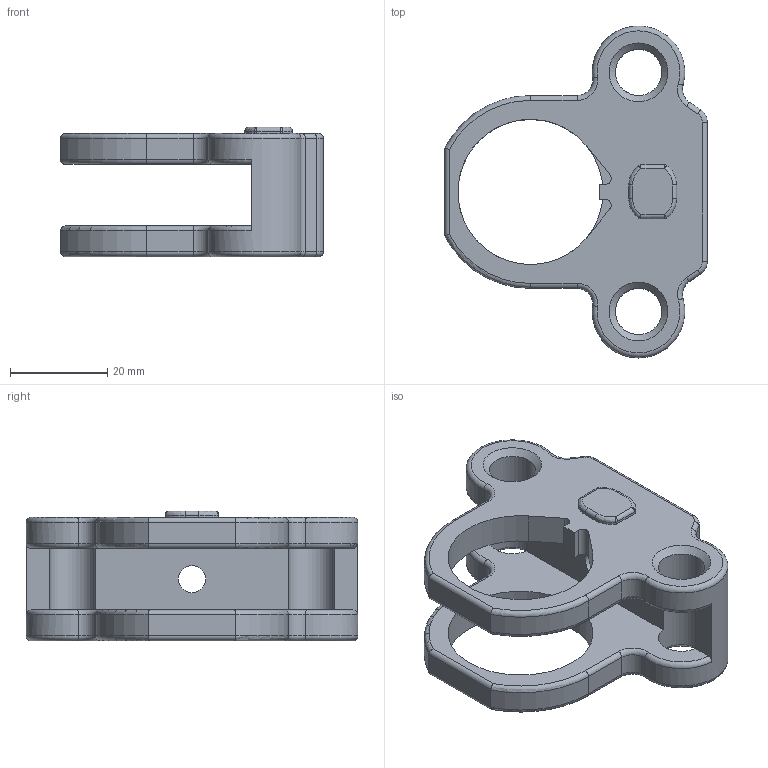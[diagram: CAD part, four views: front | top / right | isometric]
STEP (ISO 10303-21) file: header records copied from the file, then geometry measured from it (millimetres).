
FILE_DESCRIPTION (( 'STEP AP214' ), '1' );
FILE_NAME ('Lock Plate.STEP', '2014-02-12T12:48:55', ( 'elpi' ), ( '' ), 'SwSTEP 2.0', 'SolidWorks 2013', '' );
FILE_SCHEMA (( 'AUTOMOTIVE_DESIGN' ));
Length unit declared in the file: inch
Products named in the file (1): Lock Plate
Bounding box: 54.1 x 68.3 x 26.7 mm (x, y, z)
Volume: 28536 mm3; surface area: 11933.5 mm2
Topology: 1 solids, 1 shells, 123 faces, 309 edges, 182 vertices
Faces by surface type: cylinder 52, torus 32, plane 27, bspline 8, cone 4
Full cylindrical faces by diameter (mm): 5.588 x1, 9.55 x2, 11.684 x1, 29.883 x1
Entity records: 4836 total; most frequent: CARTESIAN_POINT 1936, DIRECTION 634, ORIENTED_EDGE 572, EDGE_CURVE 286, AXIS2_PLACEMENT_3D 260, VERTEX_POINT 174, EDGE_LOOP 146, CIRCLE 144
